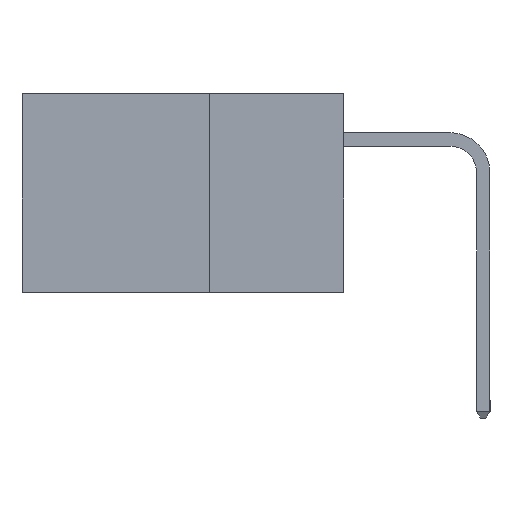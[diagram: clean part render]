
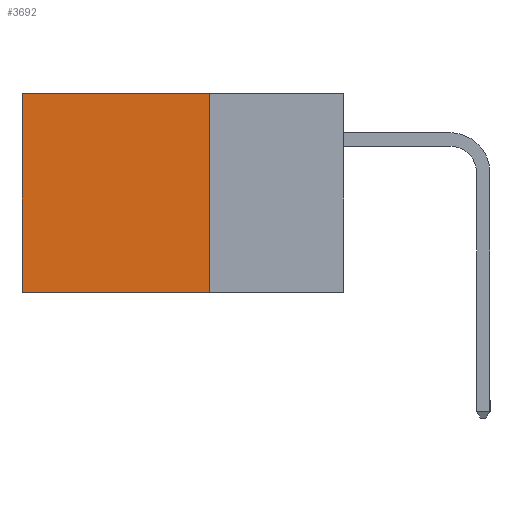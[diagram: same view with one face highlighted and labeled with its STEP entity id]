
A CAD part, left-side view. The second image highlights one B-rep face of the part: STEP entity #3692.
In plain terms, the highlighted planar face has unit normal (-1, 0, 0).
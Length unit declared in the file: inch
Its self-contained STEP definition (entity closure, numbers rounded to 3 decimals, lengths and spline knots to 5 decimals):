
#758 = LINE ( 'NONE', #15789, #14976 ) ;
#1262 = EDGE_CURVE ( 'NONE', #7606, #8454, #8513, .T. ) ;
#1585 = DIRECTION ( 'NONE',  ( 0., 0., -1. ) ) ;
#1814 = ORIENTED_EDGE ( 'NONE', *, *, #15060, .F. ) ;
#2663 = CARTESIAN_POINT ( 'NONE',  ( 0.2615, 0.6, -0.37 ) ) ;
#3684 = CARTESIAN_POINT ( 'NONE',  ( 0.2615, 0.6, 0. ) ) ;
#3692 = ADVANCED_FACE ( 'NONE', ( #7840 ), #13252, .F. ) ;
#3830 = DIRECTION ( 'NONE',  ( 0., 1., 0. ) ) ;
#5032 = VERTEX_POINT ( 'NONE', #9213 ) ;
#6250 = LINE ( 'NONE', #8667, #9894 ) ;
#6492 = DIRECTION ( 'NONE',  ( 0., 0., -1. ) ) ;
#7599 = EDGE_CURVE ( 'NONE', #5032, #11828, #15419, .T. ) ;
#7606 = VERTEX_POINT ( 'NONE', #11898 ) ;
#7840 = FACE_OUTER_BOUND ( 'NONE', #8178, .T. ) ;
#8178 = EDGE_LOOP ( 'NONE', ( #9386, #12966, #1814, #12198 ) ) ;
#8454 = VERTEX_POINT ( 'NONE', #2663 ) ;
#8513 = LINE ( 'NONE', #14827, #8937 ) ;
#8667 = CARTESIAN_POINT ( 'NONE',  ( 0.2615, 0.6, -0.37 ) ) ;
#8937 = VECTOR ( 'NONE', #3830, 39.37008 ) ;
#9213 = CARTESIAN_POINT ( 'NONE',  ( 0.2615, 0.25, 0. ) ) ;
#9386 = ORIENTED_EDGE ( 'NONE', *, *, #11859, .T. ) ;
#9894 = VECTOR ( 'NONE', #1585, 39.37008 ) ;
#9910 = AXIS2_PLACEMENT_3D ( 'NONE', #13815, #13166, #13141 ) ;
#11828 = VERTEX_POINT ( 'NONE', #3684 ) ;
#11859 = EDGE_CURVE ( 'NONE', #11828, #8454, #6250, .T. ) ;
#11898 = CARTESIAN_POINT ( 'NONE',  ( 0.2615, 0.25, -0.37 ) ) ;
#11942 = VECTOR ( 'NONE', #12067, 39.37008 ) ;
#12067 = DIRECTION ( 'NONE',  ( 0., 1., 0. ) ) ;
#12089 = CARTESIAN_POINT ( 'NONE',  ( 0.2615, 0.25, 0. ) ) ;
#12198 = ORIENTED_EDGE ( 'NONE', *, *, #7599, .T. ) ;
#12966 = ORIENTED_EDGE ( 'NONE', *, *, #1262, .F. ) ;
#13141 = DIRECTION ( 'NONE',  ( 0., 0., -1. ) ) ;
#13166 = DIRECTION ( 'NONE',  ( 1., 0., 0. ) ) ;
#13252 = PLANE ( 'NONE',  #9910 ) ;
#13815 = CARTESIAN_POINT ( 'NONE',  ( 0.2615, 0.25, -0.37 ) ) ;
#14827 = CARTESIAN_POINT ( 'NONE',  ( 0.2615, 0.25, -0.37 ) ) ;
#14976 = VECTOR ( 'NONE', #6492, 39.37008 ) ;
#15060 = EDGE_CURVE ( 'NONE', #5032, #7606, #758, .T. ) ;
#15419 = LINE ( 'NONE', #12089, #11942 ) ;
#15789 = CARTESIAN_POINT ( 'NONE',  ( 0.2615, 0.25, -0.37 ) ) ;
